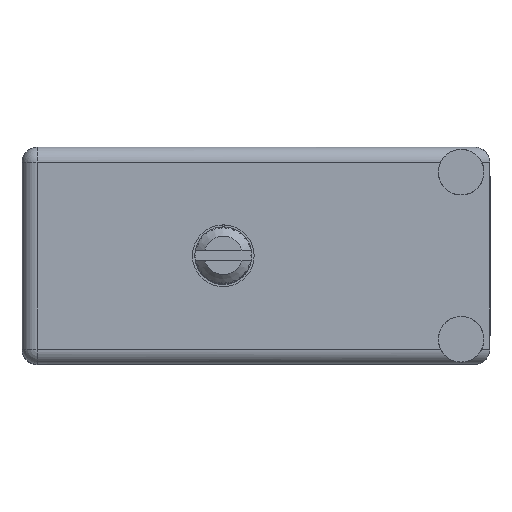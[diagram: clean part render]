
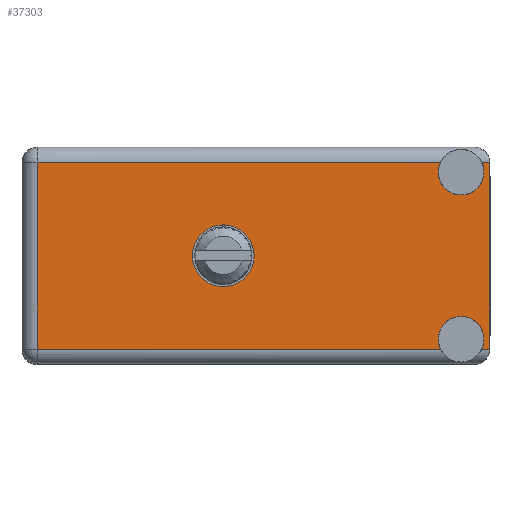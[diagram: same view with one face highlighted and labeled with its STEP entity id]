
A CAD part, top view. The second image highlights one B-rep face of the part: STEP entity #37303.
In plain terms, the highlighted face is planar.
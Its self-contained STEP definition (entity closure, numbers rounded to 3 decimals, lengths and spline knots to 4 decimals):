
#1504 = VERTEX_POINT ( 'NONE', #142696 ) ;
#3067 = ORIENTED_EDGE ( 'NONE', *, *, #92694, .T. ) ;
#6302 = EDGE_CURVE ( 'NONE', #156147, #189487, #45935, .T. ) ;
#6311 = AXIS2_PLACEMENT_3D ( 'NONE', #13584, #156815, #40539 ) ;
#6422 = DIRECTION ( 'NONE',  ( 0., 0., 1. ) ) ;
#11266 = AXIS2_PLACEMENT_3D ( 'NONE', #48328, #79056, #89686 ) ;
#12252 = CARTESIAN_POINT ( 'NONE',  ( 0.8765, 0.806, 0.3075 ) ) ;
#13010 = DIRECTION ( 'NONE',  ( 0., 0., 1. ) ) ;
#13135 = EDGE_CURVE ( 'NONE', #23459, #93437, #63975, .T. ) ;
#13584 = CARTESIAN_POINT ( 'NONE',  ( 0.7825, 0.806, -0.275 ) ) ;
#13611 = CARTESIAN_POINT ( 'NONE',  ( -0.6125, 0.806, 0.3075 ) ) ;
#15430 = CARTESIAN_POINT ( 'NONE',  ( -0.6625, 0.806, -0.3075 ) ) ;
#17352 = DIRECTION ( 'NONE',  ( -1., 0., 0. ) ) ;
#20344 = AXIS2_PLACEMENT_3D ( 'NONE', #139367, #52852, #78867 ) ;
#23459 = VERTEX_POINT ( 'NONE', #43120 ) ;
#27299 = CARTESIAN_POINT ( 'NONE',  ( -0.6625, 0.806, -0.3575 ) ) ;
#27828 = CIRCLE ( 'NONE', #6311, 0.075 ) ;
#30729 = CIRCLE ( 'NONE', #76894, 0.1015 ) ;
#32584 = EDGE_CURVE ( 'NONE', #61495, #93437, #136976, .T. ) ;
#36470 = CARTESIAN_POINT ( 'NONE',  ( 0.7825, 0.806, 0.2 ) ) ;
#36733 = CARTESIAN_POINT ( 'NONE',  ( 0.8765, 0.806, 0.3075 ) ) ;
#37303 = ADVANCED_FACE ( 'NONE', ( #58062, #115733 ), #127314, .T. ) ;
#37970 = DIRECTION ( 'NONE',  ( 0., 0., 1. ) ) ;
#40539 = DIRECTION ( 'NONE',  ( 0., 0., 1. ) ) ;
#41606 = EDGE_CURVE ( 'NONE', #189138, #1504, #124875, .T. ) ;
#42649 = VERTEX_POINT ( 'NONE', #119997 ) ;
#43120 = CARTESIAN_POINT ( 'NONE',  ( 0.8765, 0.806, -0.3075 ) ) ;
#43441 = CARTESIAN_POINT ( 'NONE',  ( 0.7825, 0.806, 0.275 ) ) ;
#43904 = LINE ( 'NONE', #12252, #58749 ) ;
#44428 = EDGE_CURVE ( 'NONE', #180619, #126613, #60648, .T. ) ;
#45935 = CIRCLE ( 'NONE', #141022, 0.075 ) ;
#47993 = CARTESIAN_POINT ( 'NONE',  ( 0.7149, 0.806, -0.3075 ) ) ;
#48328 = CARTESIAN_POINT ( 'NONE',  ( 0., 0.806, 0. ) ) ;
#49516 = ORIENTED_EDGE ( 'NONE', *, *, #44428, .T. ) ;
#52399 = CARTESIAN_POINT ( 'NONE',  ( 0.7825, 0.806, 0.275 ) ) ;
#52631 = DIRECTION ( 'NONE',  ( 1., 0., 0. ) ) ;
#52852 = DIRECTION ( 'NONE',  ( 0., 1., 0. ) ) ;
#58062 = FACE_BOUND ( 'NONE', #165319, .T. ) ;
#58189 = CARTESIAN_POINT ( 'NONE',  ( 0.8765, 0.806, 0.3575 ) ) ;
#58749 = VECTOR ( 'NONE', #113232, 39.3701 ) ;
#60648 = LINE ( 'NONE', #15430, #69190 ) ;
#61495 = VERTEX_POINT ( 'NONE', #146455 ) ;
#62173 = CARTESIAN_POINT ( 'NONE',  ( 0.7149, 0.806, 0.3075 ) ) ;
#63975 = LINE ( 'NONE', #122563, #84033 ) ;
#69190 = VECTOR ( 'NONE', #17352, 39.3701 ) ;
#75985 = VERTEX_POINT ( 'NONE', #36733 ) ;
#76894 = AXIS2_PLACEMENT_3D ( 'NONE', #168489, #150329, #109940 ) ;
#78295 = EDGE_CURVE ( 'NONE', #1504, #189138, #30729, .T. ) ;
#78867 = DIRECTION ( 'NONE',  ( 0., 0., 1. ) ) ;
#79056 = DIRECTION ( 'NONE',  ( 0., 1., 0. ) ) ;
#83736 = CARTESIAN_POINT ( 'NONE',  ( 0., 0.806, 0.1015 ) ) ;
#84033 = VECTOR ( 'NONE', #93710, 39.3701 ) ;
#86774 = EDGE_CURVE ( 'NONE', #180619, #61495, #27828, .T. ) ;
#89686 = DIRECTION ( 'NONE',  ( 0., 0., 1. ) ) ;
#90141 = EDGE_CURVE ( 'NONE', #42649, #75985, #43904, .T. ) ;
#90535 = DIRECTION ( 'NONE',  ( 0., 0., 1. ) ) ;
#92694 = EDGE_CURVE ( 'NONE', #126613, #174216, #168803, .T. ) ;
#93437 = VERTEX_POINT ( 'NONE', #100073 ) ;
#93710 = DIRECTION ( 'NONE',  ( -1., 0., 0. ) ) ;
#96981 = ORIENTED_EDGE ( 'NONE', *, *, #86774, .F. ) ;
#99485 = VECTOR ( 'NONE', #13010, 39.3701 ) ;
#100073 = CARTESIAN_POINT ( 'NONE',  ( 0.8501, 0.806, -0.3075 ) ) ;
#104765 = ORIENTED_EDGE ( 'NONE', *, *, #6302, .F. ) ;
#108176 = ORIENTED_EDGE ( 'NONE', *, *, #78295, .F. ) ;
#109940 = DIRECTION ( 'NONE',  ( 0., 0., 1. ) ) ;
#113232 = DIRECTION ( 'NONE',  ( 1., 0., 0. ) ) ;
#114784 = DIRECTION ( 'NONE',  ( -1., 0., 0. ) ) ;
#115733 = FACE_OUTER_BOUND ( 'NONE', #131700, .T. ) ;
#119997 = CARTESIAN_POINT ( 'NONE',  ( 0.8501, 0.806, 0.3075 ) ) ;
#121471 = AXIS2_PLACEMENT_3D ( 'NONE', #27299, #160837, #114784 ) ;
#121916 = LINE ( 'NONE', #151653, #142357 ) ;
#122563 = CARTESIAN_POINT ( 'NONE',  ( -0.6625, 0.806, -0.3075 ) ) ;
#124875 = CIRCLE ( 'NONE', #11266, 0.1015 ) ;
#125789 = CARTESIAN_POINT ( 'NONE',  ( -0.6125, 0.806, -0.3075 ) ) ;
#126613 = VERTEX_POINT ( 'NONE', #125789 ) ;
#127314 = PLANE ( 'NONE',  #121471 ) ;
#130256 = VECTOR ( 'NONE', #6422, 39.3701 ) ;
#131226 = LINE ( 'NONE', #58189, #99485 ) ;
#131700 = EDGE_LOOP ( 'NONE', ( #172337, #104765, #140029, #140808, #155842, #174352, #170472, #96981, #49516, #3067 ) ) ;
#136976 = CIRCLE ( 'NONE', #20344, 0.075 ) ;
#139367 = CARTESIAN_POINT ( 'NONE',  ( 0.7825, 0.806, -0.275 ) ) ;
#140000 = CARTESIAN_POINT ( 'NONE',  ( -0.6125, 0.806, -0.3575 ) ) ;
#140029 = ORIENTED_EDGE ( 'NONE', *, *, #145787, .F. ) ;
#140808 = ORIENTED_EDGE ( 'NONE', *, *, #90141, .T. ) ;
#141022 = AXIS2_PLACEMENT_3D ( 'NONE', #43441, #176065, #90535 ) ;
#142357 = VECTOR ( 'NONE', #52631, 39.3701 ) ;
#142696 = CARTESIAN_POINT ( 'NONE',  ( 0., 0.806, -0.1015 ) ) ;
#145787 = EDGE_CURVE ( 'NONE', #42649, #156147, #152151, .T. ) ;
#146455 = CARTESIAN_POINT ( 'NONE',  ( 0.7825, 0.806, -0.2 ) ) ;
#150329 = DIRECTION ( 'NONE',  ( 0., 1., 0. ) ) ;
#151653 = CARTESIAN_POINT ( 'NONE',  ( 0.8765, 0.806, 0.3075 ) ) ;
#152151 = CIRCLE ( 'NONE', #161306, 0.075 ) ;
#155842 = ORIENTED_EDGE ( 'NONE', *, *, #157931, .F. ) ;
#156147 = VERTEX_POINT ( 'NONE', #36470 ) ;
#156815 = DIRECTION ( 'NONE',  ( 0., 1., 0. ) ) ;
#157931 = EDGE_CURVE ( 'NONE', #23459, #75985, #131226, .T. ) ;
#160837 = DIRECTION ( 'NONE',  ( 0., 1., 0. ) ) ;
#161306 = AXIS2_PLACEMENT_3D ( 'NONE', #52399, #169611, #37970 ) ;
#165319 = EDGE_LOOP ( 'NONE', ( #173075, #108176 ) ) ;
#168489 = CARTESIAN_POINT ( 'NONE',  ( 0., 0.806, 0. ) ) ;
#168803 = LINE ( 'NONE', #140000, #130256 ) ;
#169611 = DIRECTION ( 'NONE',  ( 0., 1., 0. ) ) ;
#170472 = ORIENTED_EDGE ( 'NONE', *, *, #32584, .F. ) ;
#172337 = ORIENTED_EDGE ( 'NONE', *, *, #183692, .T. ) ;
#173075 = ORIENTED_EDGE ( 'NONE', *, *, #41606, .F. ) ;
#174216 = VERTEX_POINT ( 'NONE', #13611 ) ;
#174352 = ORIENTED_EDGE ( 'NONE', *, *, #13135, .T. ) ;
#176065 = DIRECTION ( 'NONE',  ( 0., 1., 0. ) ) ;
#180619 = VERTEX_POINT ( 'NONE', #47993 ) ;
#183692 = EDGE_CURVE ( 'NONE', #174216, #189487, #121916, .T. ) ;
#189138 = VERTEX_POINT ( 'NONE', #83736 ) ;
#189487 = VERTEX_POINT ( 'NONE', #62173 ) ;
